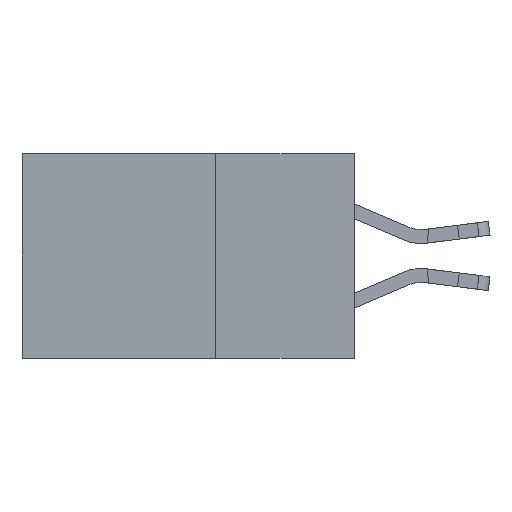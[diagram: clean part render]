
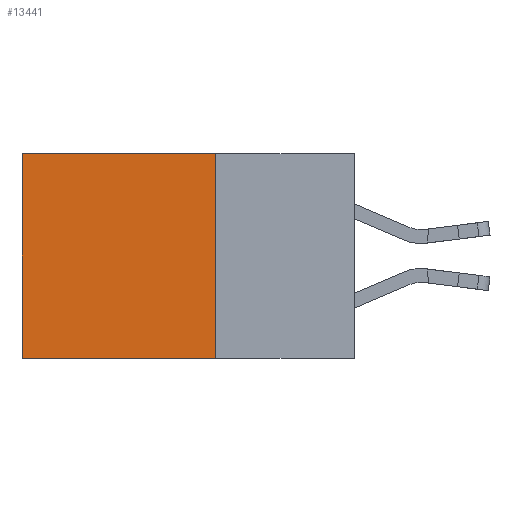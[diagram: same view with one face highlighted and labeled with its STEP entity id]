
A CAD part, left-side view. The second image highlights one B-rep face of the part: STEP entity #13441.
In plain terms, the highlighted planar face has unit normal (-1, 0, 0).
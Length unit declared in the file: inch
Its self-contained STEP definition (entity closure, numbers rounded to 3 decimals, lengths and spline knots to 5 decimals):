
#519 = VECTOR ( 'NONE', #15076, 39.37008 ) ;
#667 = CARTESIAN_POINT ( 'NONE',  ( 0.298, 0.25, -0.37 ) ) ;
#877 = FACE_OUTER_BOUND ( 'NONE', #2091, .T. ) ;
#1922 = EDGE_CURVE ( 'NONE', #12412, #9130, #2458, .T. ) ;
#2091 = EDGE_LOOP ( 'NONE', ( #3311, #5359, #2648, #17030 ) ) ;
#2458 = LINE ( 'NONE', #8458, #5858 ) ;
#2648 = ORIENTED_EDGE ( 'NONE', *, *, #1922, .F. ) ;
#3311 = ORIENTED_EDGE ( 'NONE', *, *, #4549, .T. ) ;
#4406 = CARTESIAN_POINT ( 'NONE',  ( 0.298, 0.25, 0. ) ) ;
#4549 = EDGE_CURVE ( 'NONE', #6283, #14690, #18391, .T. ) ;
#4744 = EDGE_CURVE ( 'NONE', #12412, #6283, #8494, .T. ) ;
#5359 = ORIENTED_EDGE ( 'NONE', *, *, #10941, .F. ) ;
#5858 = VECTOR ( 'NONE', #7556, 39.37008 ) ;
#6283 = VERTEX_POINT ( 'NONE', #7023 ) ;
#6916 = VECTOR ( 'NONE', #15666, 39.37008 ) ;
#7023 = CARTESIAN_POINT ( 'NONE',  ( 0.298, 0.6, 0. ) ) ;
#7317 = PLANE ( 'NONE',  #12334 ) ;
#7556 = DIRECTION ( 'NONE',  ( 0., 0., -1. ) ) ;
#8221 = LINE ( 'NONE', #667, #519 ) ;
#8458 = CARTESIAN_POINT ( 'NONE',  ( 0.298, 0.25, 0. ) ) ;
#8494 = LINE ( 'NONE', #14264, #8940 ) ;
#8738 = DIRECTION ( 'NONE',  ( 0., 0., -1. ) ) ;
#8940 = VECTOR ( 'NONE', #14089, 39.37008 ) ;
#9130 = VERTEX_POINT ( 'NONE', #12481 ) ;
#10280 = CARTESIAN_POINT ( 'NONE',  ( 0.298, 0.6, -0.37 ) ) ;
#10920 = CARTESIAN_POINT ( 'NONE',  ( 0.298, 0.25, 0. ) ) ;
#10941 = EDGE_CURVE ( 'NONE', #9130, #14690, #8221, .T. ) ;
#12334 = AXIS2_PLACEMENT_3D ( 'NONE', #4406, #17388, #8738 ) ;
#12412 = VERTEX_POINT ( 'NONE', #10920 ) ;
#12481 = CARTESIAN_POINT ( 'NONE',  ( 0.298, 0.25, -0.37 ) ) ;
#13441 = ADVANCED_FACE ( 'NONE', ( #877 ), #7317, .F. ) ;
#14089 = DIRECTION ( 'NONE',  ( 0., 1., 0. ) ) ;
#14264 = CARTESIAN_POINT ( 'NONE',  ( 0.298, 0.25, 0. ) ) ;
#14690 = VERTEX_POINT ( 'NONE', #10280 ) ;
#15076 = DIRECTION ( 'NONE',  ( 0., 1., 0. ) ) ;
#15666 = DIRECTION ( 'NONE',  ( 0., 0., -1. ) ) ;
#16277 = CARTESIAN_POINT ( 'NONE',  ( 0.298, 0.6, 0. ) ) ;
#17030 = ORIENTED_EDGE ( 'NONE', *, *, #4744, .T. ) ;
#17388 = DIRECTION ( 'NONE',  ( 1., 0., 0. ) ) ;
#18391 = LINE ( 'NONE', #16277, #6916 ) ;
